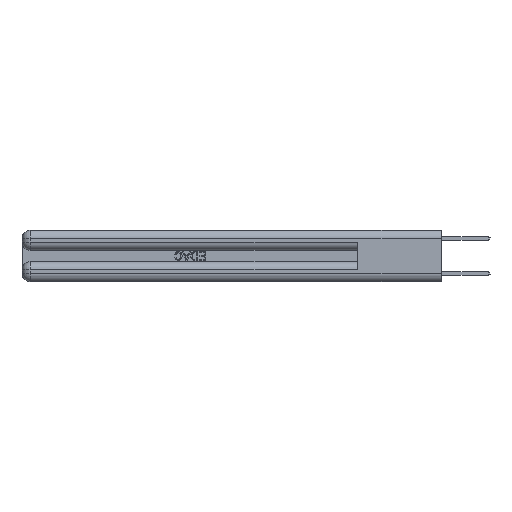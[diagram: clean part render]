
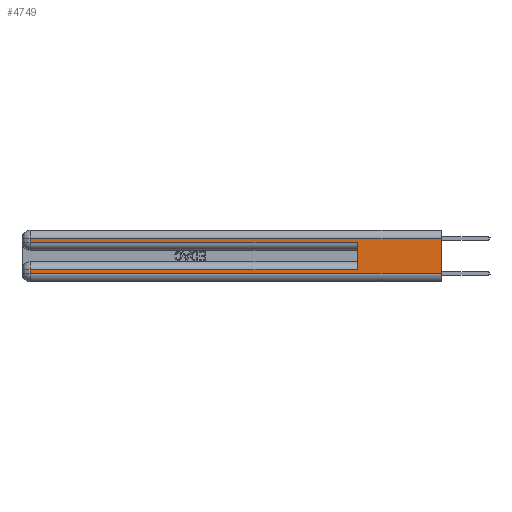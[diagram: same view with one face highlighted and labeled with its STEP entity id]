
A CAD part, left-side view. The second image highlights one B-rep face of the part: STEP entity #4749.
In plain terms, the highlighted planar face has unit normal (-1, 0, 0).
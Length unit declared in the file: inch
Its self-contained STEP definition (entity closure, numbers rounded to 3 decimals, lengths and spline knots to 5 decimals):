
#378 = EDGE_CURVE ( 'NONE', #15870, #21672, #29670, .T. ) ;
#557 = EDGE_CURVE ( 'NONE', #4140, #15227, #26310, .T. ) ;
#680 = CARTESIAN_POINT ( 'NONE',  ( 0., 0., 0.085 ) ) ;
#1278 = LINE ( 'NONE', #680, #3140 ) ;
#1836 = PLANE ( 'NONE',  #24628 ) ;
#2134 = ORIENTED_EDGE ( 'NONE', *, *, #557, .F. ) ;
#2787 = ORIENTED_EDGE ( 'NONE', *, *, #378, .T. ) ;
#3140 = VECTOR ( 'NONE', #7650, 39.37008 ) ;
#3431 = CARTESIAN_POINT ( 'NONE',  ( 0., 2.94, 0.085 ) ) ;
#4140 = VERTEX_POINT ( 'NONE', #19297 ) ;
#4749 = ADVANCED_FACE ( 'NONE', ( #15468 ), #1836, .F. ) ;
#4957 = VERTEX_POINT ( 'NONE', #15914 ) ;
#5176 = DIRECTION ( 'NONE',  ( 0., 1., 0. ) ) ;
#5825 = VECTOR ( 'NONE', #19914, 39.37008 ) ;
#6144 = CARTESIAN_POINT ( 'NONE',  ( 0., 2.94, 0.285 ) ) ;
#6694 = ORIENTED_EDGE ( 'NONE', *, *, #18857, .T. ) ;
#7562 = CARTESIAN_POINT ( 'NONE',  ( 0., 2.94, 0.31 ) ) ;
#7650 = DIRECTION ( 'NONE',  ( 0., 1., 0. ) ) ;
#8311 = EDGE_CURVE ( 'NONE', #4957, #15227, #17273, .T. ) ;
#8609 = LINE ( 'NONE', #11477, #24340 ) ;
#8649 = CARTESIAN_POINT ( 'NONE',  ( 0., 0., 0.37 ) ) ;
#8888 = CARTESIAN_POINT ( 'NONE',  ( 0., 0., 0.285 ) ) ;
#9538 = EDGE_CURVE ( 'NONE', #26079, #15870, #28953, .T. ) ;
#10874 = DIRECTION ( 'NONE',  ( 0., 0., -1. ) ) ;
#11179 = ORIENTED_EDGE ( 'NONE', *, *, #8311, .T. ) ;
#11477 = CARTESIAN_POINT ( 'NONE',  ( 0., 2.94, 0.37 ) ) ;
#13469 = CARTESIAN_POINT ( 'NONE',  ( 0., 0.6, 0.285 ) ) ;
#14506 = ORIENTED_EDGE ( 'NONE', *, *, #21058, .T. ) ;
#14745 = VERTEX_POINT ( 'NONE', #3431 ) ;
#14961 = CARTESIAN_POINT ( 'NONE',  ( 0., 0., 0.06 ) ) ;
#15227 = VERTEX_POINT ( 'NONE', #14961 ) ;
#15468 = FACE_OUTER_BOUND ( 'NONE', #25539, .T. ) ;
#15870 = VERTEX_POINT ( 'NONE', #6144 ) ;
#15914 = CARTESIAN_POINT ( 'NONE',  ( 0., 2.94, 0.06 ) ) ;
#16716 = LINE ( 'NONE', #23382, #18153 ) ;
#17273 = LINE ( 'NONE', #28946, #25441 ) ;
#17423 = DIRECTION ( 'NONE',  ( 0., 0., -1. ) ) ;
#18120 = EDGE_CURVE ( 'NONE', #4140, #26079, #28372, .T. ) ;
#18128 = DIRECTION ( 'NONE',  ( 0., -1., 0. ) ) ;
#18153 = VECTOR ( 'NONE', #25985, 39.37008 ) ;
#18286 = VERTEX_POINT ( 'NONE', #26832 ) ;
#18293 = ORIENTED_EDGE ( 'NONE', *, *, #18120, .T. ) ;
#18857 = EDGE_CURVE ( 'NONE', #14745, #4957, #8609, .T. ) ;
#18964 = VECTOR ( 'NONE', #5176, 39.37008 ) ;
#19297 = CARTESIAN_POINT ( 'NONE',  ( 0., 0., 0.31 ) ) ;
#19914 = DIRECTION ( 'NONE',  ( 0., 0., -1. ) ) ;
#21058 = EDGE_CURVE ( 'NONE', #18286, #14745, #1278, .T. ) ;
#21524 = DIRECTION ( 'NONE',  ( 0., -1., 0. ) ) ;
#21672 = VERTEX_POINT ( 'NONE', #13469 ) ;
#21784 = VECTOR ( 'NONE', #18128, 39.37008 ) ;
#21815 = CARTESIAN_POINT ( 'NONE',  ( 0., 2.94, 0.37 ) ) ;
#22751 = EDGE_CURVE ( 'NONE', #18286, #21672, #16716, .T. ) ;
#23382 = CARTESIAN_POINT ( 'NONE',  ( 0., 0.6, 0.145 ) ) ;
#24026 = ORIENTED_EDGE ( 'NONE', *, *, #9538, .T. ) ;
#24340 = VECTOR ( 'NONE', #10874, 39.37008 ) ;
#24562 = DIRECTION ( 'NONE',  ( 0., 0., -1. ) ) ;
#24628 = AXIS2_PLACEMENT_3D ( 'NONE', #8649, #29426, #24562 ) ;
#25441 = VECTOR ( 'NONE', #21524, 39.37008 ) ;
#25539 = EDGE_LOOP ( 'NONE', ( #2134, #18293, #24026, #2787, #29033, #14506, #6694, #11179 ) ) ;
#25798 = CARTESIAN_POINT ( 'NONE',  ( 0., 0., 0.31 ) ) ;
#25985 = DIRECTION ( 'NONE',  ( 0., 0., 1. ) ) ;
#26079 = VERTEX_POINT ( 'NONE', #7562 ) ;
#26310 = LINE ( 'NONE', #26744, #5825 ) ;
#26744 = CARTESIAN_POINT ( 'NONE',  ( 0., 0., 0.37 ) ) ;
#26832 = CARTESIAN_POINT ( 'NONE',  ( 0., 0.6, 0.085 ) ) ;
#27029 = VECTOR ( 'NONE', #17423, 39.37008 ) ;
#28372 = LINE ( 'NONE', #25798, #18964 ) ;
#28946 = CARTESIAN_POINT ( 'NONE',  ( 0., 0., 0.06 ) ) ;
#28953 = LINE ( 'NONE', #21815, #27029 ) ;
#29033 = ORIENTED_EDGE ( 'NONE', *, *, #22751, .F. ) ;
#29426 = DIRECTION ( 'NONE',  ( 1., 0., 0. ) ) ;
#29670 = LINE ( 'NONE', #8888, #21784 ) ;
